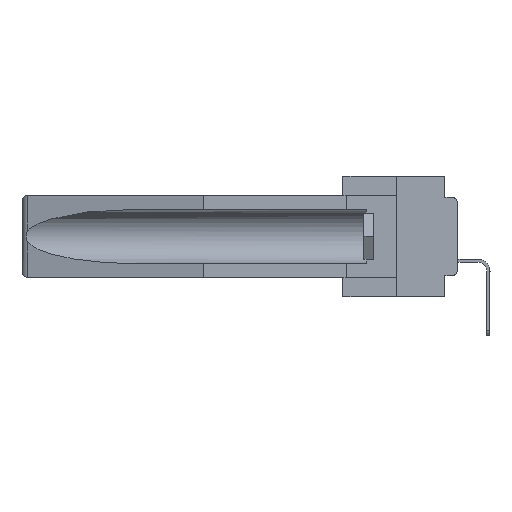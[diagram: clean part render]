
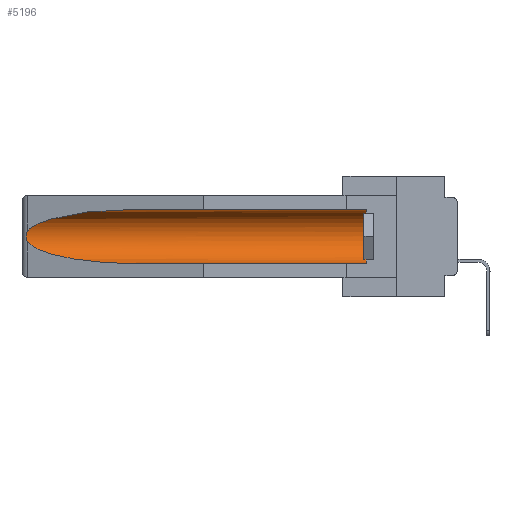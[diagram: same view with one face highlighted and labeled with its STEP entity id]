
A CAD part, left-side view. The second image highlights one B-rep face of the part: STEP entity #5196.
In plain terms, the highlighted cylindrical face has radius 2.857 mm (diameter 5.715 mm), a partial arc.
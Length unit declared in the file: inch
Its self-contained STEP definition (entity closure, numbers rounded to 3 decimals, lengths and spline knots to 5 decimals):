
#95 = EDGE_CURVE ( 'NONE', #6712, #21377, #19379, .T. ) ;
#354 = VECTOR ( 'NONE', #21668, 39.37008 ) ;
#1381 = CARTESIAN_POINT ( 'NONE',  ( 0.26537, 1.52718, -0.14972 ) ) ;
#2043 = DIRECTION ( 'NONE',  ( 0., 0., 1. ) ) ;
#2809 = CARTESIAN_POINT ( 'NONE',  ( 0.155, 0.126, -0.059 ) ) ;
#3055 = DIRECTION ( 'NONE',  ( 0., 0., 1. ) ) ;
#4390 = CARTESIAN_POINT ( 'NONE',  ( 0.2675, 1.53308, -0.16763 ) ) ;
#4626 = FACE_OUTER_BOUND ( 'NONE', #12138, .T. ) ;
#5196 = ADVANCED_FACE ( 'NONE', ( #4626 ), #15795, .F. ) ;
#6712 = VERTEX_POINT ( 'NONE', #19623 ) ;
#7292 = DIRECTION ( 'NONE',  ( 0., 1., 0. ) ) ;
#7630 = EDGE_CURVE ( 'NONE', #21377, #22895, #20284, .T. ) ;
#7793 = CARTESIAN_POINT ( 'NONE',  ( 0.155, -0.30754, -0.284 ) ) ;
#8208 = CARTESIAN_POINT ( 'NONE',  ( 0.26537, 1.52718, -0.14972 ) ) ;
#8416 = CARTESIAN_POINT ( 'NONE',  ( 0.25451, 1.48313, -0.09465 ) ) ;
#8910 = CARTESIAN_POINT ( 'NONE',  ( 0.26654, 1.53092, -0.15636 ) ) ;
#9105 = CARTESIAN_POINT ( 'NONE',  ( 0.155, 1.07973, -0.284 ) ) ;
#9304 = CARTESIAN_POINT ( 'NONE',  ( 0.26537, 1.52718, -0.14972 ) ) ;
#10239 = EDGE_CURVE ( 'NONE', #22895, #18278, #22382, .T. ) ;
#10522 = AXIS2_PLACEMENT_3D ( 'NONE', #14593, #19244, #3055 ) ;
#11113 = LINE ( 'NONE', #7793, #354 ) ;
#11190 = CARTESIAN_POINT ( 'NONE',  ( 0.2675, 1.53308, -0.17534 ) ) ;
#11554 = DIRECTION ( 'NONE',  ( 0., -1., 0. ) ) ;
#12138 = EDGE_LOOP ( 'NONE', ( #25772, #26164, #23511, #27654, #15961, #18577 ) ) ;
#12997 = CARTESIAN_POINT ( 'NONE',  ( 0.21114, 1.30732, -0.059 ) ) ;
#13462 = CARTESIAN_POINT ( 'NONE',  ( 0.155, 0.126, -0.1715 ) ) ;
#13596 = CARTESIAN_POINT ( 'NONE',  ( 0.25451, 1.48313, -0.24835 ) ) ;
#13602 = CARTESIAN_POINT ( 'NONE',  ( 0.26597, 1.5296, -0.19026 ) ) ;
#14287 =( BOUNDED_CURVE ( )  B_SPLINE_CURVE ( 3, ( #20881, #13596, #23065, #9105 ),
 .UNSPECIFIED., .F., .F. ) 
 B_SPLINE_CURVE_WITH_KNOTS ( ( 4, 4 ),
 ( 0.1948, 1.5708 ),
 .UNSPECIFIED. ) 
 CURVE ( )  GEOMETRIC_REPRESENTATION_ITEM ( )  RATIONAL_B_SPLINE_CURVE ( ( 1., 0.848, 0.848, 1. ) ) 
 REPRESENTATION_ITEM ( '' )  );
#14593 = CARTESIAN_POINT ( 'NONE',  ( 0.155, -0.30754, -0.1715 ) ) ;
#15795 = CYLINDRICAL_SURFACE ( 'NONE', #10522, 0.1125 ) ;
#15961 = ORIENTED_EDGE ( 'NONE', *, *, #95, .T. ) ;
#16342 = CARTESIAN_POINT ( 'NONE',  ( 0.155, -0.30754, -0.059 ) ) ;
#16908 = EDGE_CURVE ( 'NONE', #6712, #24579, #11113, .T. ) ;
#16975 = VERTEX_POINT ( 'NONE', #22132 ) ;
#17365 = CARTESIAN_POINT ( 'NONE',  ( 0.155, 1.07973, -0.059 ) ) ;
#18056 = CARTESIAN_POINT ( 'NONE',  ( 0.26597, 1.52961, -0.15275 ) ) ;
#18103 = VECTOR ( 'NONE', #7292, 39.37008 ) ;
#18278 = VERTEX_POINT ( 'NONE', #8208 ) ;
#18577 = ORIENTED_EDGE ( 'NONE', *, *, #7630, .T. ) ;
#19244 = DIRECTION ( 'NONE',  ( 0., 1., 0. ) ) ;
#19347 = CARTESIAN_POINT ( 'NONE',  ( 0.155, 1.07973, -0.059 ) ) ;
#19379 = CIRCLE ( 'NONE', #21604, 0.1125 ) ;
#19623 = CARTESIAN_POINT ( 'NONE',  ( 0.155, 0.126, -0.284 ) ) ;
#20097 = EDGE_CURVE ( 'NONE', #16975, #24579, #14287, .T. ) ;
#20284 = LINE ( 'NONE', #16342, #18103 ) ;
#20881 = CARTESIAN_POINT ( 'NONE',  ( 0.26537, 1.52718, -0.19328 ) ) ;
#21377 = VERTEX_POINT ( 'NONE', #2809 ) ;
#21604 = AXIS2_PLACEMENT_3D ( 'NONE', #13462, #11554, #2043 ) ;
#21664 = CARTESIAN_POINT ( 'NONE',  ( 0.155, 1.07973, -0.284 ) ) ;
#21668 = DIRECTION ( 'NONE',  ( 0., 1., 0. ) ) ;
#22132 = CARTESIAN_POINT ( 'NONE',  ( 0.26537, 1.52718, -0.19328 ) ) ;
#22382 =( BOUNDED_CURVE ( )  B_SPLINE_CURVE ( 3, ( #17365, #12997, #8416, #1381 ),
 .UNSPECIFIED., .F., .T. ) 
 B_SPLINE_CURVE_WITH_KNOTS ( ( 4, 4 ),
 ( 4.71239, 6.08839 ),
 .UNSPECIFIED. ) 
 CURVE ( )  GEOMETRIC_REPRESENTATION_ITEM ( )  RATIONAL_B_SPLINE_CURVE ( ( 1., 0.848, 0.848, 1. ) ) 
 REPRESENTATION_ITEM ( '' )  );
#22767 = CARTESIAN_POINT ( 'NONE',  ( 0.2673, 1.53269, -0.17917 ) ) ;
#22895 = VERTEX_POINT ( 'NONE', #19347 ) ;
#23065 = CARTESIAN_POINT ( 'NONE',  ( 0.21114, 1.30732, -0.284 ) ) ;
#23511 = ORIENTED_EDGE ( 'NONE', *, *, #20097, .T. ) ;
#24579 = VERTEX_POINT ( 'NONE', #21664 ) ;
#24959 = CARTESIAN_POINT ( 'NONE',  ( 0.2673, 1.5327, -0.16383 ) ) ;
#25047 = CARTESIAN_POINT ( 'NONE',  ( 0.26655, 1.53094, -0.18657 ) ) ;
#25772 = ORIENTED_EDGE ( 'NONE', *, *, #10239, .T. ) ;
#26164 = ORIENTED_EDGE ( 'NONE', *, *, #27901, .T. ) ;
#27654 = ORIENTED_EDGE ( 'NONE', *, *, #16908, .F. ) ;
#27901 = EDGE_CURVE ( 'NONE', #18278, #16975, #29364, .T. ) ;
#29364 = B_SPLINE_CURVE_WITH_KNOTS ( 'NONE', 3,
 ( #9304, #18056, #8910, #24959, #4390, #11190, #22767, #25047, #13602, #29673 ),
 .UNSPECIFIED., .F., .F.,
 ( 4, 2, 2, 2, 4 ),
 ( 0., 0.00029, 0.00058, 0.00087, 0.00117 ),
 .UNSPECIFIED. ) ;
#29673 = CARTESIAN_POINT ( 'NONE',  ( 0.26537, 1.52718, -0.19328 ) ) ;
